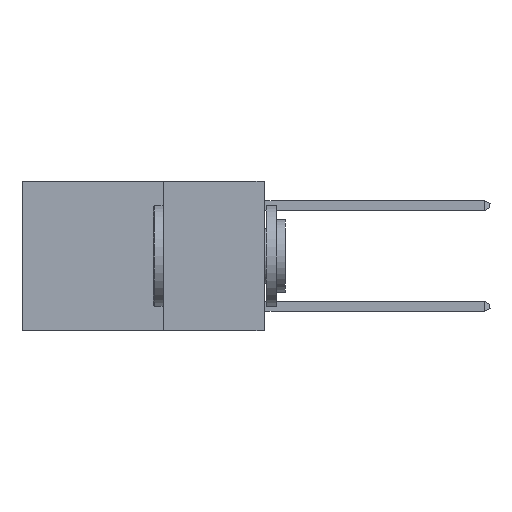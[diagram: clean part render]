
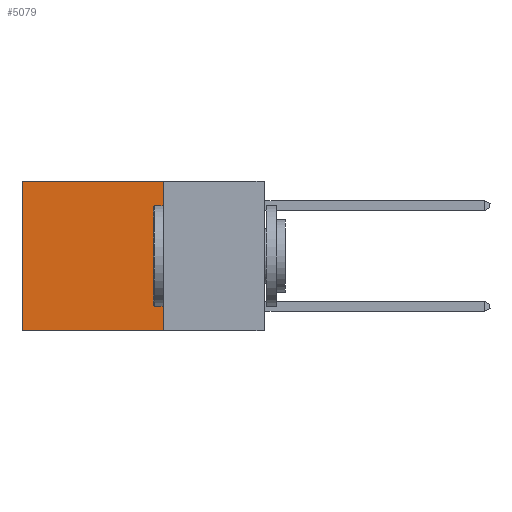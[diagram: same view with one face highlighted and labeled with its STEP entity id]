
A CAD part, left-side view. The second image highlights one B-rep face of the part: STEP entity #5079.
In plain terms, the highlighted planar face has unit normal (-1, 0, 0).
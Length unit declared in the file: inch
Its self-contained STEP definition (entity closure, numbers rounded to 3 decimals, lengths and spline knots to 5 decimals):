
#1537 = CARTESIAN_POINT ( 'NONE',  ( 0.2625, 0.6, -0.37 ) ) ;
#1891 = DIRECTION ( 'NONE',  ( 0., 0., -1. ) ) ;
#2000 = LINE ( 'NONE', #7561, #12782 ) ;
#2122 = ORIENTED_EDGE ( 'NONE', *, *, #3102, .T. ) ;
#2172 = LINE ( 'NONE', #22660, #13552 ) ;
#2722 = CARTESIAN_POINT ( 'NONE',  ( 0.2625, 0.25, 0. ) ) ;
#2923 = ORIENTED_EDGE ( 'NONE', *, *, #13759, .F. ) ;
#3102 = EDGE_CURVE ( 'NONE', #16173, #10578, #2000, .T. ) ;
#3810 = ORIENTED_EDGE ( 'NONE', *, *, #6601, .T. ) ;
#5079 = ADVANCED_FACE ( 'NONE', ( #9768 ), #19346, .F. ) ;
#5095 = CARTESIAN_POINT ( 'NONE',  ( 0.2625, 0.25, 0. ) ) ;
#6219 = EDGE_LOOP ( 'NONE', ( #2122, #2923, #9182, #3810 ) ) ;
#6601 = EDGE_CURVE ( 'NONE', #20445, #16173, #16792, .T. ) ;
#6914 = EDGE_CURVE ( 'NONE', #20445, #18889, #21463, .T. ) ;
#7561 = CARTESIAN_POINT ( 'NONE',  ( 0.2625, 0.6, 0. ) ) ;
#9182 = ORIENTED_EDGE ( 'NONE', *, *, #6914, .F. ) ;
#9768 = FACE_OUTER_BOUND ( 'NONE', #6219, .T. ) ;
#10578 = VERTEX_POINT ( 'NONE', #1537 ) ;
#11248 = DIRECTION ( 'NONE',  ( 0., 1., 0. ) ) ;
#11275 = VECTOR ( 'NONE', #12958, 39.37008 ) ;
#12782 = VECTOR ( 'NONE', #1891, 39.37008 ) ;
#12958 = DIRECTION ( 'NONE',  ( 0., 0., -1. ) ) ;
#13552 = VECTOR ( 'NONE', #17244, 39.37008 ) ;
#13656 = VECTOR ( 'NONE', #11248, 39.37008 ) ;
#13759 = EDGE_CURVE ( 'NONE', #18889, #10578, #2172, .T. ) ;
#15444 = DIRECTION ( 'NONE',  ( 0., 0., -1. ) ) ;
#15685 = CARTESIAN_POINT ( 'NONE',  ( 0.2625, 0.6, 0. ) ) ;
#16173 = VERTEX_POINT ( 'NONE', #15685 ) ;
#16554 = CARTESIAN_POINT ( 'NONE',  ( 0.2625, 0.25, 0. ) ) ;
#16792 = LINE ( 'NONE', #5095, #13656 ) ;
#17244 = DIRECTION ( 'NONE',  ( 0., 1., 0. ) ) ;
#18889 = VERTEX_POINT ( 'NONE', #22968 ) ;
#19346 = PLANE ( 'NONE',  #19491 ) ;
#19491 = AXIS2_PLACEMENT_3D ( 'NONE', #21327, #23066, #15444 ) ;
#20445 = VERTEX_POINT ( 'NONE', #16554 ) ;
#21327 = CARTESIAN_POINT ( 'NONE',  ( 0.2625, 0.25, 0. ) ) ;
#21463 = LINE ( 'NONE', #2722, #11275 ) ;
#22660 = CARTESIAN_POINT ( 'NONE',  ( 0.2625, 0.25, -0.37 ) ) ;
#22968 = CARTESIAN_POINT ( 'NONE',  ( 0.2625, 0.25, -0.37 ) ) ;
#23066 = DIRECTION ( 'NONE',  ( 1., 0., 0. ) ) ;
